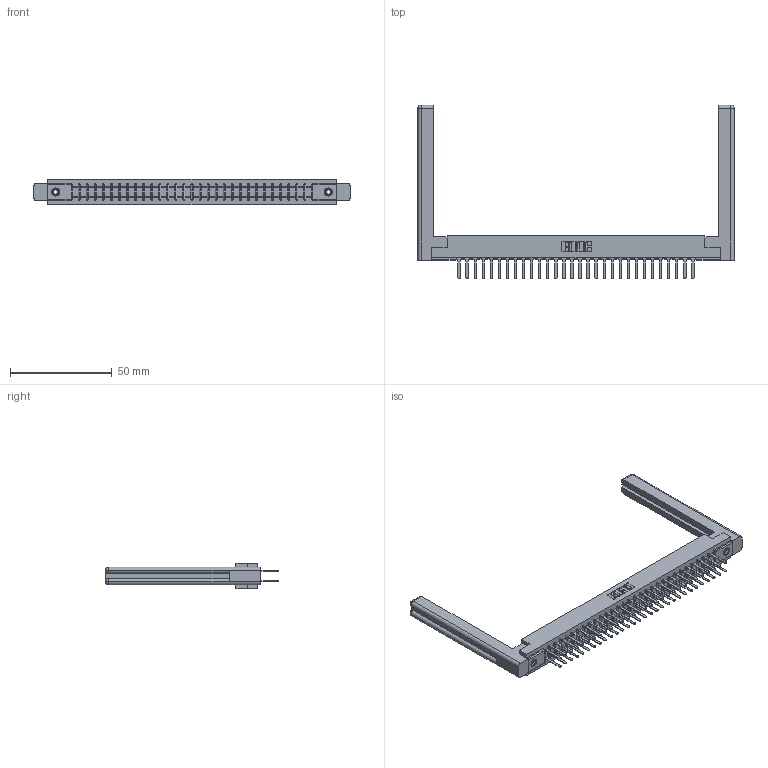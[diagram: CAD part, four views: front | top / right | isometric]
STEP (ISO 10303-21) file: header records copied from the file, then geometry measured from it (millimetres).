
FILE_DESCRIPTION (( 'STEP AP203' ), '1' );
FILE_NAME ('307-060-422-258.STEP', '2020-09-30T13:51:03', ( '' ), ( '' ), 'SwSTEP 2.0', 'SolidWorks 2020', '' );
FILE_SCHEMA (( 'CONFIG_CONTROL_DESIGN' ));
Length unit declared in the file: inch
Products named in the file (5): 345-250-001_345-250-001-102; 307 Part_.156 Dia Mounting Holes; 307-060-422-258; 307-290-001_522; 307-220-058
Assembly tree (65 placements, depth 2):
  307-060-422-258
    307 Part_.156 Dia Mounting Holes
    307-290-001_522  x60
    307-220-058  x2
    345-250-001_345-250-001-102  x2
Bounding box: 155.5 x 85.42 x 12.7 mm (x, y, z)
Volume: 23709.1 mm3; surface area: 25591.8 mm2
Topology: 65 solids, 65 shells, 3051 faces, 8477 edges, 5474 vertices
Faces by surface type: plane 2014, cylinder 951, sphere 62, torus 12, cone 12
Entity records: 30759 total; most frequent: CARTESIAN_POINT 5053, ORIENTED_EDGE 4948, DIRECTION 4912, EDGE_CURVE 2474, VECTOR 1890, LINE 1890, VERTEX_POINT 1598, AXIS2_PLACEMENT_3D 1511
